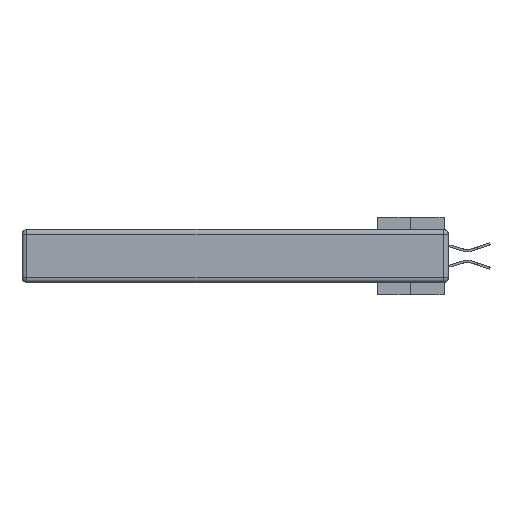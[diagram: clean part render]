
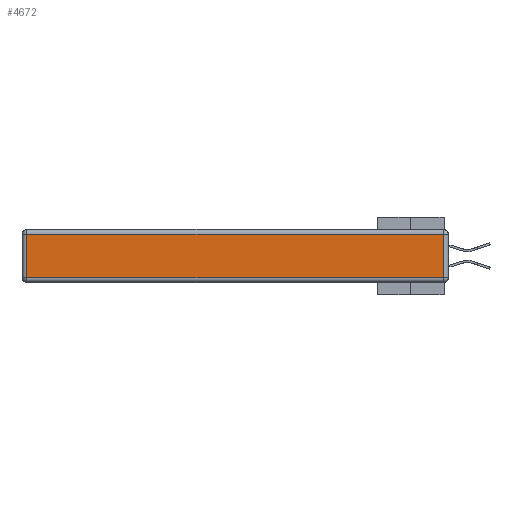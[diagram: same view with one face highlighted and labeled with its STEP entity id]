
A CAD part, left-side view. The second image highlights one B-rep face of the part: STEP entity #4672.
In plain terms, the highlighted planar face has unit normal (-1, 0, 0).
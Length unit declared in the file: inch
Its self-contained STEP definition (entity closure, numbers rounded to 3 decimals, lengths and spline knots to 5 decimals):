
#3676 = ORIENTED_EDGE ( 'NONE', *, *, #4215, .T. ) ;
#3966 = DIRECTION ( 'NONE',  ( 0., 0., 1. ) ) ;
#4215 = EDGE_CURVE ( 'NONE', #8661, #31160, #38061, .T. ) ;
#4672 = ADVANCED_FACE ( 'NONE', ( #29981 ), #31246, .T. ) ;
#4987 = VECTOR ( 'NONE', #33083, 39.37008 ) ;
#6000 = VERTEX_POINT ( 'NONE', #14220 ) ;
#8661 = VERTEX_POINT ( 'NONE', #33244 ) ;
#8671 = EDGE_CURVE ( 'NONE', #29368, #8661, #8891, .T. ) ;
#8891 = LINE ( 'NONE', #24150, #14579 ) ;
#11227 = EDGE_LOOP ( 'NONE', ( #37532, #17649, #26039, #3676 ) ) ;
#13321 = EDGE_CURVE ( 'NONE', #31160, #6000, #14241, .T. ) ;
#13831 = CARTESIAN_POINT ( 'NONE',  ( 0., 2.72, -0.343 ) ) ;
#14220 = CARTESIAN_POINT ( 'NONE',  ( 0., 0.03, -0.313 ) ) ;
#14241 = LINE ( 'NONE', #25774, #27507 ) ;
#14579 = VECTOR ( 'NONE', #18171, 39.37008 ) ;
#17649 = ORIENTED_EDGE ( 'NONE', *, *, #31126, .T. ) ;
#18171 = DIRECTION ( 'NONE',  ( 0., 1., 0. ) ) ;
#18854 = CARTESIAN_POINT ( 'NONE',  ( 0., 0.03, -0.03 ) ) ;
#20626 = LINE ( 'NONE', #21077, #4987 ) ;
#21077 = CARTESIAN_POINT ( 'NONE',  ( 0., 0.03, -0.343 ) ) ;
#21347 = AXIS2_PLACEMENT_3D ( 'NONE', #31494, #28599, #3966 ) ;
#21992 = VECTOR ( 'NONE', #37652, 39.37008 ) ;
#24150 = CARTESIAN_POINT ( 'NONE',  ( 0., 2.75, -0.03 ) ) ;
#25638 = DIRECTION ( 'NONE',  ( 0., -1., 0. ) ) ;
#25774 = CARTESIAN_POINT ( 'NONE',  ( 0., 0., -0.313 ) ) ;
#26039 = ORIENTED_EDGE ( 'NONE', *, *, #8671, .T. ) ;
#27507 = VECTOR ( 'NONE', #25638, 39.37008 ) ;
#28599 = DIRECTION ( 'NONE',  ( -1., 0., 0. ) ) ;
#29368 = VERTEX_POINT ( 'NONE', #18854 ) ;
#29981 = FACE_OUTER_BOUND ( 'NONE', #11227, .T. ) ;
#31126 = EDGE_CURVE ( 'NONE', #6000, #29368, #20626, .T. ) ;
#31160 = VERTEX_POINT ( 'NONE', #36396 ) ;
#31246 = PLANE ( 'NONE',  #21347 ) ;
#31494 = CARTESIAN_POINT ( 'NONE',  ( 0., 0., -0.343 ) ) ;
#33083 = DIRECTION ( 'NONE',  ( 0., 0., 1. ) ) ;
#33244 = CARTESIAN_POINT ( 'NONE',  ( 0., 2.72, -0.03 ) ) ;
#36396 = CARTESIAN_POINT ( 'NONE',  ( 0., 2.72, -0.313 ) ) ;
#37532 = ORIENTED_EDGE ( 'NONE', *, *, #13321, .T. ) ;
#37652 = DIRECTION ( 'NONE',  ( 0., 0., -1. ) ) ;
#38061 = LINE ( 'NONE', #13831, #21992 ) ;
